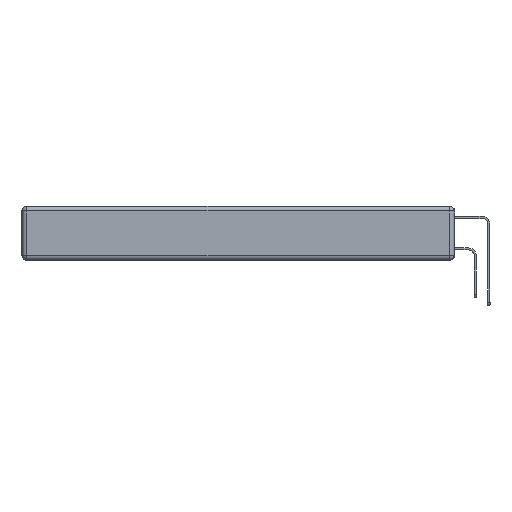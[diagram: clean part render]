
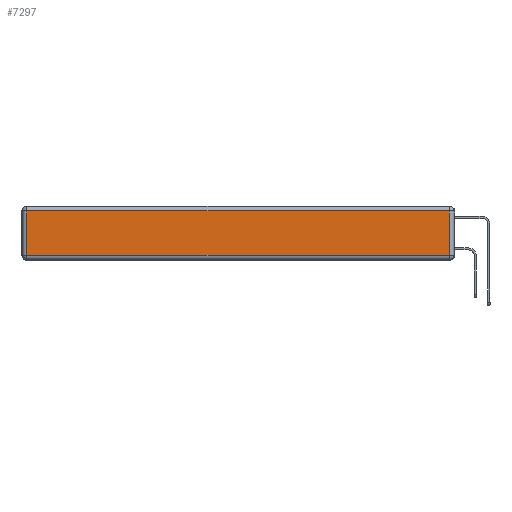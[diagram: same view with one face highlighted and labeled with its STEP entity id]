
A CAD part, left-side view. The second image highlights one B-rep face of the part: STEP entity #7297.
In plain terms, the highlighted planar face has unit normal (-1, 0, 0).
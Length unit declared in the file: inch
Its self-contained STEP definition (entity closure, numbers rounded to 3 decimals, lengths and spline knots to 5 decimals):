
#20 = LINE ( 'NONE', #15220, #12015 ) ;
#286 = CARTESIAN_POINT ( 'NONE',  ( 0., 0., -0.343 ) ) ;
#346 = EDGE_CURVE ( 'NONE', #4287, #19815, #15624, .T. ) ;
#386 = DIRECTION ( 'NONE',  ( -1., 0., 0. ) ) ;
#854 = CARTESIAN_POINT ( 'NONE',  ( 0., 0.03, -0.03 ) ) ;
#2014 = DIRECTION ( 'NONE',  ( 0., -1., 0. ) ) ;
#2663 = VECTOR ( 'NONE', #3960, 39.37008 ) ;
#3666 = VERTEX_POINT ( 'NONE', #854 ) ;
#3809 = PLANE ( 'NONE',  #5650 ) ;
#3960 = DIRECTION ( 'NONE',  ( 0., 0., 1. ) ) ;
#4287 = VERTEX_POINT ( 'NONE', #18493 ) ;
#5208 = DIRECTION ( 'NONE',  ( 0., 0., -1. ) ) ;
#5650 = AXIS2_PLACEMENT_3D ( 'NONE', #286, #386, #7319 ) ;
#5733 = EDGE_CURVE ( 'NONE', #3666, #4287, #20, .T. ) ;
#7297 = ADVANCED_FACE ( 'NONE', ( #19337 ), #3809, .T. ) ;
#7319 = DIRECTION ( 'NONE',  ( 0., 0., 1. ) ) ;
#10421 = CARTESIAN_POINT ( 'NONE',  ( 0., 2.72, -0.343 ) ) ;
#10996 = ORIENTED_EDGE ( 'NONE', *, *, #13518, .T. ) ;
#12015 = VECTOR ( 'NONE', #15456, 39.37008 ) ;
#12580 = CARTESIAN_POINT ( 'NONE',  ( 0., 0.03, -0.343 ) ) ;
#12646 = LINE ( 'NONE', #16054, #15285 ) ;
#13518 = EDGE_CURVE ( 'NONE', #13902, #3666, #15636, .T. ) ;
#13902 = VERTEX_POINT ( 'NONE', #21864 ) ;
#14785 = CARTESIAN_POINT ( 'NONE',  ( 0., 2.72, -0.313 ) ) ;
#15220 = CARTESIAN_POINT ( 'NONE',  ( 0., 2.75, -0.03 ) ) ;
#15285 = VECTOR ( 'NONE', #2014, 39.37008 ) ;
#15456 = DIRECTION ( 'NONE',  ( 0., 1., 0. ) ) ;
#15477 = VECTOR ( 'NONE', #5208, 39.37008 ) ;
#15624 = LINE ( 'NONE', #10421, #15477 ) ;
#15636 = LINE ( 'NONE', #12580, #2663 ) ;
#16054 = CARTESIAN_POINT ( 'NONE',  ( 0., 0., -0.313 ) ) ;
#18493 = CARTESIAN_POINT ( 'NONE',  ( 0., 2.72, -0.03 ) ) ;
#19211 = EDGE_LOOP ( 'NONE', ( #19468, #10996, #19861, #20048 ) ) ;
#19337 = FACE_OUTER_BOUND ( 'NONE', #19211, .T. ) ;
#19468 = ORIENTED_EDGE ( 'NONE', *, *, #19598, .T. ) ;
#19598 = EDGE_CURVE ( 'NONE', #19815, #13902, #12646, .T. ) ;
#19815 = VERTEX_POINT ( 'NONE', #14785 ) ;
#19861 = ORIENTED_EDGE ( 'NONE', *, *, #5733, .T. ) ;
#20048 = ORIENTED_EDGE ( 'NONE', *, *, #346, .T. ) ;
#21864 = CARTESIAN_POINT ( 'NONE',  ( 0., 0.03, -0.313 ) ) ;
